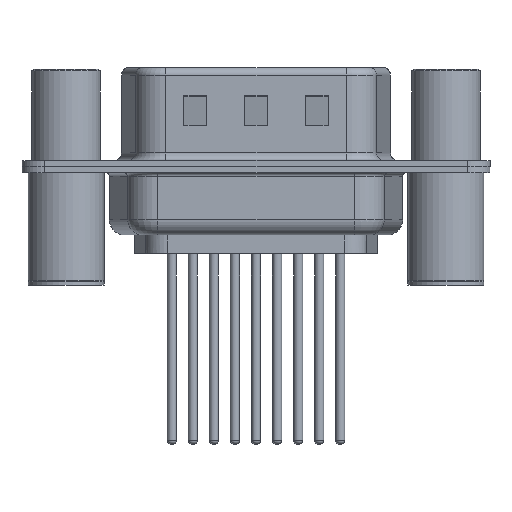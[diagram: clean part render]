
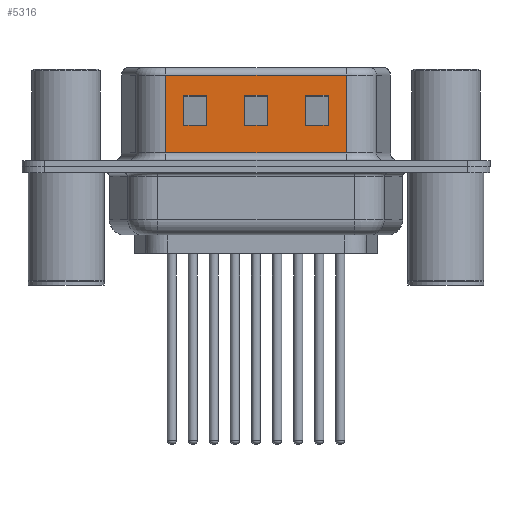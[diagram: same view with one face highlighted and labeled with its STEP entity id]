
A CAD part, front view. The second image highlights one B-rep face of the part: STEP entity #5316.
In plain terms, the highlighted planar face has unit normal (0, -1, 0).
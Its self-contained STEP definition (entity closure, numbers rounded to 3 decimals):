
#29 = VERTEX_POINT ( 'NONE', #4891 ) ;
#46 = VERTEX_POINT ( 'NONE', #9887 ) ;
#93 = VERTEX_POINT ( 'NONE', #2216 ) ;
#708 = LINE ( 'NONE', #6573, #5403 ) ;
#828 = ORIENTED_EDGE ( 'NONE', *, *, #2302, .T. ) ;
#944 = CARTESIAN_POINT ( 'NONE',  ( 15.75, -4.55, 6.52 ) ) ;
#1260 = DIRECTION ( 'NONE',  ( 0., 0., -1. ) ) ;
#1337 = LINE ( 'NONE', #12316, #11889 ) ;
#1348 = LINE ( 'NONE', #12634, #15078 ) ;
#1500 = ORIENTED_EDGE ( 'NONE', *, *, #7346, .T. ) ;
#1514 = EDGE_CURVE ( 'NONE', #10616, #8048, #2970, .T. ) ;
#1535 = VECTOR ( 'NONE', #3539, 1000. ) ;
#1635 = VECTOR ( 'NONE', #7936, 1000. ) ;
#1812 = EDGE_CURVE ( 'NONE', #10843, #9921, #3984, .T. ) ;
#1833 = CARTESIAN_POINT ( 'NONE',  ( 13.25, -4.55, 6.52 ) ) ;
#1958 = LINE ( 'NONE', #12638, #2307 ) ;
#2087 = CARTESIAN_POINT ( 'NONE',  ( 9.25, -4.55, 6.52 ) ) ;
#2216 = CARTESIAN_POINT ( 'NONE',  ( 18.451, -4.55, 6.02 ) ) ;
#2254 = FACE_OUTER_BOUND ( 'NONE', #13562, .T. ) ;
#2302 = EDGE_CURVE ( 'NONE', #14412, #4361, #13466, .T. ) ;
#2307 = VECTOR ( 'NONE', #6914, 1000. ) ;
#2426 = PLANE ( 'NONE',  #12180 ) ;
#2475 = CARTESIAN_POINT ( 'NONE',  ( 18.451, -4.55, 4.705 ) ) ;
#2499 = CARTESIAN_POINT ( 'NONE',  ( 18.451, -4.55, 6.52 ) ) ;
#2678 = VERTEX_POINT ( 'NONE', #9083 ) ;
#2970 = LINE ( 'NONE', #5245, #1635 ) ;
#3035 = EDGE_CURVE ( 'NONE', #5299, #2678, #1337, .T. ) ;
#3104 = EDGE_CURVE ( 'NONE', #93, #7837, #11026, .T. ) ;
#3414 = CARTESIAN_POINT ( 'NONE',  ( 18.451, -4.55, 0.9 ) ) ;
#3528 = EDGE_CURVE ( 'NONE', #15636, #8837, #12431, .T. ) ;
#3539 = DIRECTION ( 'NONE',  ( -1., 0., 0. ) ) ;
#3727 = EDGE_CURVE ( 'NONE', #8048, #7837, #708, .T. ) ;
#3821 = EDGE_CURVE ( 'NONE', #4361, #10843, #4832, .T. ) ;
#3835 = DIRECTION ( 'NONE',  ( -1., 0., 0. ) ) ;
#3984 = LINE ( 'NONE', #8888, #10006 ) ;
#3988 = CARTESIAN_POINT ( 'NONE',  ( 7.75, -4.55, 4.705 ) ) ;
#4099 = CARTESIAN_POINT ( 'NONE',  ( 22.451, -4.55, 4.705 ) ) ;
#4170 = EDGE_CURVE ( 'NONE', #46, #29, #7863, .T. ) ;
#4361 = VERTEX_POINT ( 'NONE', #5728 ) ;
#4445 = DIRECTION ( 'NONE',  ( 0., 0., -1. ) ) ;
#4518 = EDGE_LOOP ( 'NONE', ( #6698, #13484, #15722, #11828 ) ) ;
#4611 = VECTOR ( 'NONE', #11471, 1000. ) ;
#4731 = CARTESIAN_POINT ( 'NONE',  ( 18.451, -4.55, 6.02 ) ) ;
#4809 = DIRECTION ( 'NONE',  ( 0., 0., -1. ) ) ;
#4832 = LINE ( 'NONE', #5748, #1535 ) ;
#4858 = ORIENTED_EDGE ( 'NONE', *, *, #3727, .T. ) ;
#4891 = CARTESIAN_POINT ( 'NONE',  ( 17.25, -4.55, 4.705 ) ) ;
#4997 = DIRECTION ( 'NONE',  ( 1., 0., 0. ) ) ;
#5245 = CARTESIAN_POINT ( 'NONE',  ( 6.549, -4.55, 6.52 ) ) ;
#5299 = VERTEX_POINT ( 'NONE', #11239 ) ;
#5316 = ADVANCED_FACE ( 'NONE', ( #14943, #12528, #13408, #2254 ), #2426, .F. ) ;
#5403 = VECTOR ( 'NONE', #5516, 1000. ) ;
#5466 = ORIENTED_EDGE ( 'NONE', *, *, #7014, .T. ) ;
#5516 = DIRECTION ( 'NONE',  ( 1., 0., 0. ) ) ;
#5728 = CARTESIAN_POINT ( 'NONE',  ( 9.25, -4.55, 2.705 ) ) ;
#5748 = CARTESIAN_POINT ( 'NONE',  ( 14.451, -4.55, 2.705 ) ) ;
#5845 = EDGE_CURVE ( 'NONE', #2678, #10157, #1958, .T. ) ;
#5955 = VECTOR ( 'NONE', #4997, 1000. ) ;
#6115 = DIRECTION ( 'NONE',  ( -1., 0., 0. ) ) ;
#6135 = LINE ( 'NONE', #944, #10446 ) ;
#6419 = VECTOR ( 'NONE', #12885, 1000. ) ;
#6477 = ORIENTED_EDGE ( 'NONE', *, *, #3104, .F. ) ;
#6573 = CARTESIAN_POINT ( 'NONE',  ( 18.451, -4.55, 0.9 ) ) ;
#6698 = ORIENTED_EDGE ( 'NONE', *, *, #14684, .T. ) ;
#6914 = DIRECTION ( 'NONE',  ( 0., 0., 1. ) ) ;
#7014 = EDGE_CURVE ( 'NONE', #29, #15636, #1348, .T. ) ;
#7116 = CARTESIAN_POINT ( 'NONE',  ( 6.549, -4.55, 6.02 ) ) ;
#7346 = EDGE_CURVE ( 'NONE', #93, #10616, #15637, .T. ) ;
#7388 = DIRECTION ( 'NONE',  ( 0., 1., 0. ) ) ;
#7473 = CARTESIAN_POINT ( 'NONE',  ( 15.75, -4.55, 2.705 ) ) ;
#7790 = CARTESIAN_POINT ( 'NONE',  ( 9.25, -4.55, 4.705 ) ) ;
#7837 = VERTEX_POINT ( 'NONE', #3414 ) ;
#7863 = LINE ( 'NONE', #4099, #15025 ) ;
#7932 = ORIENTED_EDGE ( 'NONE', *, *, #8204, .T. ) ;
#7936 = DIRECTION ( 'NONE',  ( 0., 0., -1. ) ) ;
#7953 = LINE ( 'NONE', #12847, #9574 ) ;
#8048 = VERTEX_POINT ( 'NONE', #13738 ) ;
#8204 = EDGE_CURVE ( 'NONE', #9921, #14412, #7953, .T. ) ;
#8596 = DIRECTION ( 'NONE',  ( 0., 0., 1. ) ) ;
#8718 = DIRECTION ( 'NONE',  ( 0., 0., 1. ) ) ;
#8837 = VERTEX_POINT ( 'NONE', #7473 ) ;
#8839 = LINE ( 'NONE', #2475, #5955 ) ;
#8888 = CARTESIAN_POINT ( 'NONE',  ( 7.75, -4.55, 6.52 ) ) ;
#9017 = VECTOR ( 'NONE', #4445, 1000. ) ;
#9083 = CARTESIAN_POINT ( 'NONE',  ( 11.75, -4.55, 2.705 ) ) ;
#9163 = CARTESIAN_POINT ( 'NONE',  ( 7.75, -4.55, 2.705 ) ) ;
#9238 = LINE ( 'NONE', #1833, #6419 ) ;
#9289 = EDGE_LOOP ( 'NONE', ( #828, #14627, #13822, #7932 ) ) ;
#9574 = VECTOR ( 'NONE', #9683, 1000. ) ;
#9683 = DIRECTION ( 'NONE',  ( 1., 0., 0. ) ) ;
#9730 = VERTEX_POINT ( 'NONE', #11332 ) ;
#9887 = CARTESIAN_POINT ( 'NONE',  ( 15.75, -4.55, 4.705 ) ) ;
#9921 = VERTEX_POINT ( 'NONE', #3988 ) ;
#9995 = ORIENTED_EDGE ( 'NONE', *, *, #4170, .T. ) ;
#10006 = VECTOR ( 'NONE', #8718, 1000. ) ;
#10157 = VERTEX_POINT ( 'NONE', #13503 ) ;
#10159 = ORIENTED_EDGE ( 'NONE', *, *, #1514, .T. ) ;
#10446 = VECTOR ( 'NONE', #8596, 1000. ) ;
#10616 = VERTEX_POINT ( 'NONE', #7116 ) ;
#10843 = VERTEX_POINT ( 'NONE', #9163 ) ;
#10993 = DIRECTION ( 'NONE',  ( 0., 0., 1. ) ) ;
#11026 = LINE ( 'NONE', #15962, #15778 ) ;
#11239 = CARTESIAN_POINT ( 'NONE',  ( 13.25, -4.55, 2.705 ) ) ;
#11332 = CARTESIAN_POINT ( 'NONE',  ( 13.25, -4.55, 4.705 ) ) ;
#11448 = CARTESIAN_POINT ( 'NONE',  ( 17.25, -4.55, 2.705 ) ) ;
#11471 = DIRECTION ( 'NONE',  ( -1., 0., 0. ) ) ;
#11734 = VECTOR ( 'NONE', #6115, 1000. ) ;
#11817 = EDGE_CURVE ( 'NONE', #8837, #46, #6135, .T. ) ;
#11828 = ORIENTED_EDGE ( 'NONE', *, *, #5845, .T. ) ;
#11889 = VECTOR ( 'NONE', #3835, 1000. ) ;
#12180 = AXIS2_PLACEMENT_3D ( 'NONE', #2499, #7388, #10993 ) ;
#12316 = CARTESIAN_POINT ( 'NONE',  ( 18.451, -4.55, 2.705 ) ) ;
#12431 = LINE ( 'NONE', #15872, #4611 ) ;
#12528 = FACE_BOUND ( 'NONE', #13340, .T. ) ;
#12634 = CARTESIAN_POINT ( 'NONE',  ( 17.25, -4.55, 6.52 ) ) ;
#12638 = CARTESIAN_POINT ( 'NONE',  ( 11.75, -4.55, 6.52 ) ) ;
#12742 = DIRECTION ( 'NONE',  ( 1., 0., 0. ) ) ;
#12847 = CARTESIAN_POINT ( 'NONE',  ( 14.451, -4.55, 4.705 ) ) ;
#12885 = DIRECTION ( 'NONE',  ( 0., 0., -1. ) ) ;
#13340 = EDGE_LOOP ( 'NONE', ( #5466, #15772, #15463, #9995 ) ) ;
#13408 = FACE_BOUND ( 'NONE', #4518, .T. ) ;
#13466 = LINE ( 'NONE', #2087, #9017 ) ;
#13473 = EDGE_CURVE ( 'NONE', #9730, #5299, #9238, .T. ) ;
#13484 = ORIENTED_EDGE ( 'NONE', *, *, #13473, .T. ) ;
#13503 = CARTESIAN_POINT ( 'NONE',  ( 11.75, -4.55, 4.705 ) ) ;
#13562 = EDGE_LOOP ( 'NONE', ( #6477, #1500, #10159, #4858 ) ) ;
#13738 = CARTESIAN_POINT ( 'NONE',  ( 6.549, -4.55, 0.9 ) ) ;
#13822 = ORIENTED_EDGE ( 'NONE', *, *, #1812, .T. ) ;
#14412 = VERTEX_POINT ( 'NONE', #7790 ) ;
#14627 = ORIENTED_EDGE ( 'NONE', *, *, #3821, .T. ) ;
#14684 = EDGE_CURVE ( 'NONE', #10157, #9730, #8839, .T. ) ;
#14943 = FACE_BOUND ( 'NONE', #9289, .T. ) ;
#15025 = VECTOR ( 'NONE', #12742, 1000. ) ;
#15078 = VECTOR ( 'NONE', #1260, 1000. ) ;
#15463 = ORIENTED_EDGE ( 'NONE', *, *, #11817, .T. ) ;
#15636 = VERTEX_POINT ( 'NONE', #11448 ) ;
#15637 = LINE ( 'NONE', #4731, #11734 ) ;
#15722 = ORIENTED_EDGE ( 'NONE', *, *, #3035, .T. ) ;
#15772 = ORIENTED_EDGE ( 'NONE', *, *, #3528, .T. ) ;
#15778 = VECTOR ( 'NONE', #4809, 1000. ) ;
#15872 = CARTESIAN_POINT ( 'NONE',  ( 22.451, -4.55, 2.705 ) ) ;
#15962 = CARTESIAN_POINT ( 'NONE',  ( 18.451, -4.55, 6.52 ) ) ;
